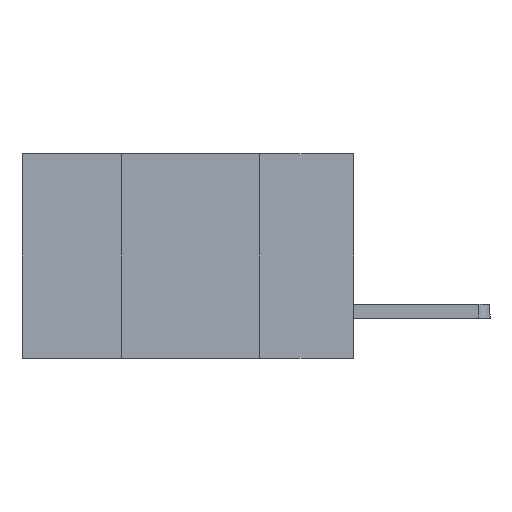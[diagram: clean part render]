
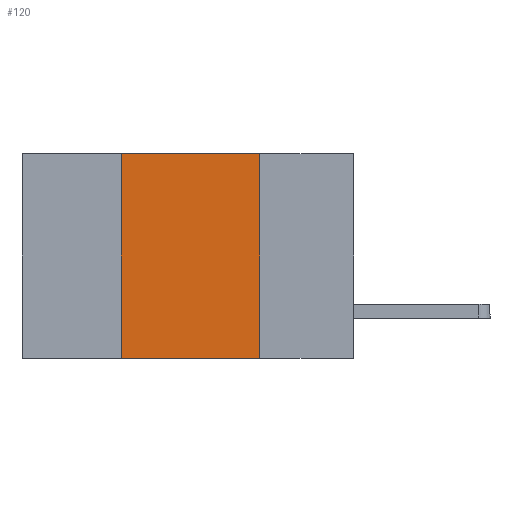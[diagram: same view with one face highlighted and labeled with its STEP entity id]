
A CAD part, left-side view. The second image highlights one B-rep face of the part: STEP entity #120.
In plain terms, the highlighted planar face has unit normal (-1, 0, 0).
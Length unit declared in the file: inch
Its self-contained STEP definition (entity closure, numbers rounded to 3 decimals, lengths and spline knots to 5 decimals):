
#120 = ADVANCED_FACE ( 'NONE', ( #3289 ), #2587, .F. ) ;
#402 = VECTOR ( 'NONE', #816, 39.37008 ) ;
#648 = AXIS2_PLACEMENT_3D ( 'NONE', #2485, #2370, #2327 ) ;
#816 = DIRECTION ( 'NONE',  ( 0., 0., 1. ) ) ;
#1986 = EDGE_LOOP ( 'NONE', ( #8639, #4559, #4991, #4844 ) ) ;
#2327 = DIRECTION ( 'NONE',  ( 0., 0., -1. ) ) ;
#2370 = DIRECTION ( 'NONE',  ( 1., 0., 0. ) ) ;
#2485 = CARTESIAN_POINT ( 'NONE',  ( 0., 0.6, 0. ) ) ;
#2535 = VERTEX_POINT ( 'NONE', #5128 ) ;
#2587 = PLANE ( 'NONE',  #648 ) ;
#2622 = EDGE_CURVE ( 'NONE', #9838, #2535, #8430, .T. ) ;
#3058 = EDGE_CURVE ( 'NONE', #4969, #3067, #8697, .T. ) ;
#3067 = VERTEX_POINT ( 'NONE', #11055 ) ;
#3220 = DIRECTION ( 'NONE',  ( 0., -1., 0. ) ) ;
#3289 = FACE_OUTER_BOUND ( 'NONE', #1986, .T. ) ;
#3448 = CARTESIAN_POINT ( 'NONE',  ( 0., 0.6, -0.37 ) ) ;
#4074 = CARTESIAN_POINT ( 'NONE',  ( 0., 0.17, 0. ) ) ;
#4079 = VECTOR ( 'NONE', #9466, 39.37008 ) ;
#4328 = CARTESIAN_POINT ( 'NONE',  ( 0., 0.42, 0. ) ) ;
#4333 = CARTESIAN_POINT ( 'NONE',  ( 0., 0.6, 0. ) ) ;
#4559 = ORIENTED_EDGE ( 'NONE', *, *, #3058, .F. ) ;
#4844 = ORIENTED_EDGE ( 'NONE', *, *, #2622, .T. ) ;
#4969 = VERTEX_POINT ( 'NONE', #4328 ) ;
#4991 = ORIENTED_EDGE ( 'NONE', *, *, #8577, .F. ) ;
#5128 = CARTESIAN_POINT ( 'NONE',  ( 0., 0.17, -0.37 ) ) ;
#5956 = VECTOR ( 'NONE', #10814, 39.37008 ) ;
#6161 = VECTOR ( 'NONE', #3220, 39.37008 ) ;
#6568 = EDGE_CURVE ( 'NONE', #3067, #2535, #8234, .T. ) ;
#7903 = CARTESIAN_POINT ( 'NONE',  ( 0., 0.42, -0.37 ) ) ;
#8234 = LINE ( 'NONE', #4074, #5956 ) ;
#8430 = LINE ( 'NONE', #3448, #6161 ) ;
#8577 = EDGE_CURVE ( 'NONE', #9838, #4969, #9722, .T. ) ;
#8639 = ORIENTED_EDGE ( 'NONE', *, *, #6568, .F. ) ;
#8697 = LINE ( 'NONE', #4333, #4079 ) ;
#9466 = DIRECTION ( 'NONE',  ( 0., -1., 0. ) ) ;
#9722 = LINE ( 'NONE', #10336, #402 ) ;
#9838 = VERTEX_POINT ( 'NONE', #7903 ) ;
#10336 = CARTESIAN_POINT ( 'NONE',  ( 0., 0.42, 0. ) ) ;
#10814 = DIRECTION ( 'NONE',  ( 0., 0., -1. ) ) ;
#11055 = CARTESIAN_POINT ( 'NONE',  ( 0., 0.17, 0. ) ) ;
